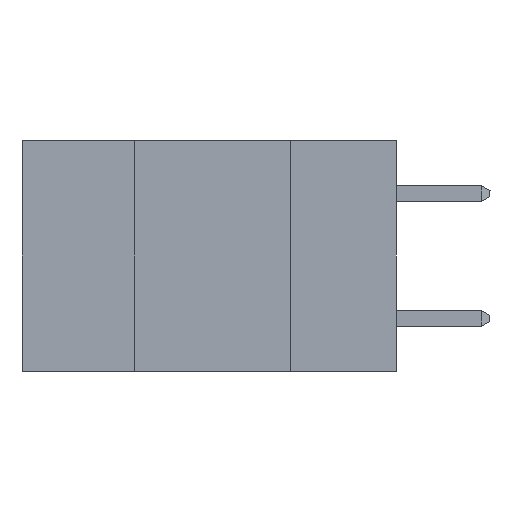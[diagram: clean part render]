
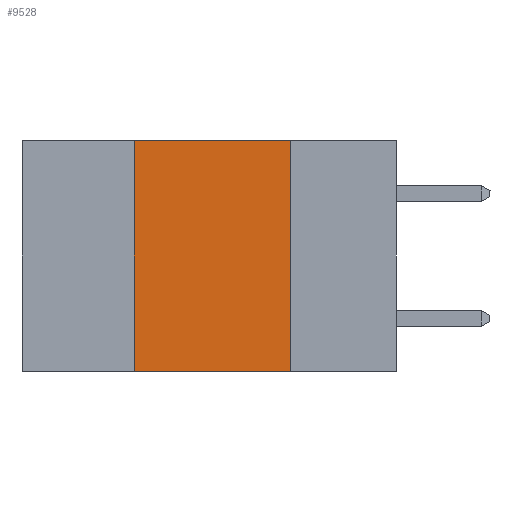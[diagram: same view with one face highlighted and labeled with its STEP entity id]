
A CAD part, left-side view. The second image highlights one B-rep face of the part: STEP entity #9528.
In plain terms, the highlighted planar face has unit normal (-1, 0, 0).
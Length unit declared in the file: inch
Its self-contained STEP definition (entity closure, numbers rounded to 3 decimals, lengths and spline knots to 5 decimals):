
#584 = AXIS2_PLACEMENT_3D ( 'NONE', #14471, #3908, #12224 ) ;
#1764 = VERTEX_POINT ( 'NONE', #11400 ) ;
#1780 = FACE_OUTER_BOUND ( 'NONE', #3398, .T. ) ;
#3398 = EDGE_LOOP ( 'NONE', ( #11346, #9004, #3686, #10834 ) ) ;
#3491 = CARTESIAN_POINT ( 'NONE',  ( 0., 0.6, -0.37 ) ) ;
#3686 = ORIENTED_EDGE ( 'NONE', *, *, #11226, .F. ) ;
#3845 = DIRECTION ( 'NONE',  ( 0., -1., 0. ) ) ;
#3908 = DIRECTION ( 'NONE',  ( 1., 0., 0. ) ) ;
#5363 = EDGE_CURVE ( 'NONE', #1764, #5451, #6789, .T. ) ;
#5372 = DIRECTION ( 'NONE',  ( 0., 0., -1. ) ) ;
#5451 = VERTEX_POINT ( 'NONE', #6741 ) ;
#5642 = VERTEX_POINT ( 'NONE', #7100 ) ;
#5677 = EDGE_CURVE ( 'NONE', #5642, #5451, #8657, .T. ) ;
#5858 = EDGE_CURVE ( 'NONE', #13115, #1764, #14944, .T. ) ;
#6027 = VECTOR ( 'NONE', #3845, 39.37008 ) ;
#6404 = VECTOR ( 'NONE', #5372, 39.37008 ) ;
#6741 = CARTESIAN_POINT ( 'NONE',  ( 0., 0.17, -0.37 ) ) ;
#6789 = LINE ( 'NONE', #12450, #6404 ) ;
#7100 = CARTESIAN_POINT ( 'NONE',  ( 0., 0.42, -0.37 ) ) ;
#8657 = LINE ( 'NONE', #3491, #14427 ) ;
#9004 = ORIENTED_EDGE ( 'NONE', *, *, #5858, .F. ) ;
#9123 = CARTESIAN_POINT ( 'NONE',  ( 0., 0.42, 0. ) ) ;
#9528 = ADVANCED_FACE ( 'NONE', ( #1780 ), #11076, .F. ) ;
#9551 = DIRECTION ( 'NONE',  ( 0., -1., 0. ) ) ;
#9557 = CARTESIAN_POINT ( 'NONE',  ( 0., 0.42, 0. ) ) ;
#10744 = DIRECTION ( 'NONE',  ( 0., 0., 1. ) ) ;
#10834 = ORIENTED_EDGE ( 'NONE', *, *, #5677, .T. ) ;
#11023 = CARTESIAN_POINT ( 'NONE',  ( 0., 0.6, 0. ) ) ;
#11076 = PLANE ( 'NONE',  #584 ) ;
#11226 = EDGE_CURVE ( 'NONE', #5642, #13115, #15106, .T. ) ;
#11346 = ORIENTED_EDGE ( 'NONE', *, *, #5363, .F. ) ;
#11400 = CARTESIAN_POINT ( 'NONE',  ( 0., 0.17, 0. ) ) ;
#12095 = VECTOR ( 'NONE', #10744, 39.37008 ) ;
#12224 = DIRECTION ( 'NONE',  ( 0., 0., -1. ) ) ;
#12450 = CARTESIAN_POINT ( 'NONE',  ( 0., 0.17, 0. ) ) ;
#13115 = VERTEX_POINT ( 'NONE', #9123 ) ;
#14427 = VECTOR ( 'NONE', #9551, 39.37008 ) ;
#14471 = CARTESIAN_POINT ( 'NONE',  ( 0., 0.6, 0. ) ) ;
#14944 = LINE ( 'NONE', #11023, #6027 ) ;
#15106 = LINE ( 'NONE', #9557, #12095 ) ;
